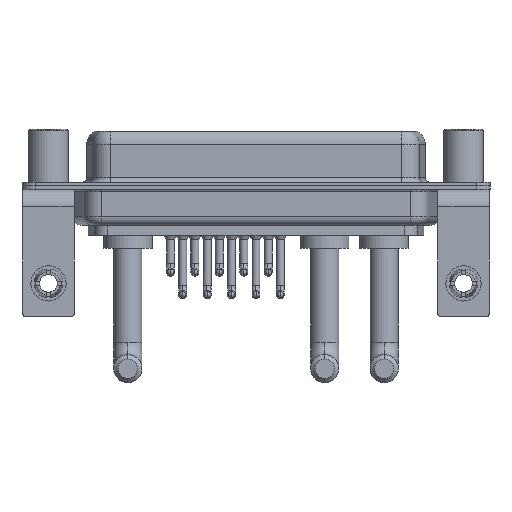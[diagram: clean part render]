
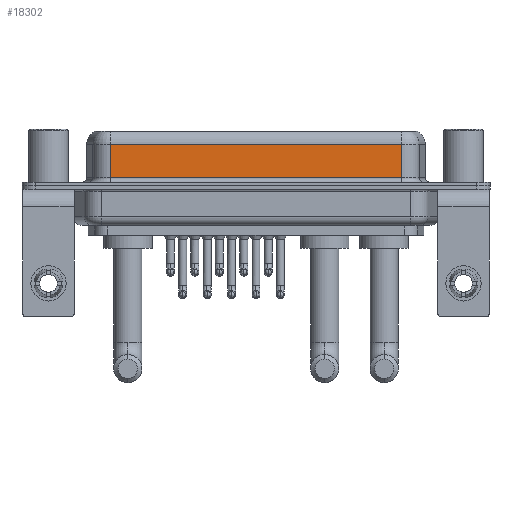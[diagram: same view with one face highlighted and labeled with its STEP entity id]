
A CAD part, front view. The second image highlights one B-rep face of the part: STEP entity #18302.
In plain terms, the highlighted planar face has unit normal (0, -1, 0).
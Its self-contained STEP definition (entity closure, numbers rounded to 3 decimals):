
#898 = EDGE_CURVE ( 'NONE', #4275, #22912, #19926, .T. ) ;
#1198 = FACE_OUTER_BOUND ( 'NONE', #8461, .T. ) ;
#2179 = EDGE_CURVE ( 'NONE', #14506, #22912, #13624, .T. ) ;
#3720 = CARTESIAN_POINT ( 'NONE',  ( 40.037, -3.95, 0.9 ) ) ;
#4275 = VERTEX_POINT ( 'NONE', #19622 ) ;
#4609 = VECTOR ( 'NONE', #14231, 1000. ) ;
#4819 = ORIENTED_EDGE ( 'NONE', *, *, #17110, .T. ) ;
#5041 = DIRECTION ( 'NONE',  ( 0., 0., -1. ) ) ;
#5207 = LINE ( 'NONE', #13895, #4609 ) ;
#5889 = CARTESIAN_POINT ( 'NONE',  ( 40.037, -3.95, 4.65 ) ) ;
#6322 = LINE ( 'NONE', #20639, #19572 ) ;
#6610 = DIRECTION ( 'NONE',  ( 0., 1., 0. ) ) ;
#6916 = DIRECTION ( 'NONE',  ( 1., 0., 0. ) ) ;
#7011 = VERTEX_POINT ( 'NONE', #16318 ) ;
#7277 = EDGE_CURVE ( 'NONE', #14506, #7011, #6322, .T. ) ;
#8328 = VECTOR ( 'NONE', #6916, 1000. ) ;
#8355 = CARTESIAN_POINT ( 'NONE',  ( 40.037, -3.95, 6.4 ) ) ;
#8461 = EDGE_LOOP ( 'NONE', ( #10611, #22834, #4819, #16038 ) ) ;
#10611 = ORIENTED_EDGE ( 'NONE', *, *, #2179, .F. ) ;
#11840 = DIRECTION ( 'NONE',  ( -1., 0., 0. ) ) ;
#13624 = LINE ( 'NONE', #21115, #14077 ) ;
#13895 = CARTESIAN_POINT ( 'NONE',  ( 7.013, -3.95, 6.4 ) ) ;
#14077 = VECTOR ( 'NONE', #5041, 1000. ) ;
#14231 = DIRECTION ( 'NONE',  ( 0., 0., -1. ) ) ;
#14506 = VERTEX_POINT ( 'NONE', #5889 ) ;
#15546 = AXIS2_PLACEMENT_3D ( 'NONE', #8355, #6610, #15631 ) ;
#15631 = DIRECTION ( 'NONE',  ( 0., 0., 1. ) ) ;
#16038 = ORIENTED_EDGE ( 'NONE', *, *, #898, .T. ) ;
#16318 = CARTESIAN_POINT ( 'NONE',  ( 7.013, -3.95, 4.65 ) ) ;
#17110 = EDGE_CURVE ( 'NONE', #7011, #4275, #5207, .T. ) ;
#17606 = CARTESIAN_POINT ( 'NONE',  ( 40.037, -3.95, 0.9 ) ) ;
#18302 = ADVANCED_FACE ( 'NONE', ( #1198 ), #19605, .F. ) ;
#19572 = VECTOR ( 'NONE', #11840, 1000. ) ;
#19605 = PLANE ( 'NONE',  #15546 ) ;
#19622 = CARTESIAN_POINT ( 'NONE',  ( 7.013, -3.95, 0.9 ) ) ;
#19926 = LINE ( 'NONE', #3720, #8328 ) ;
#20639 = CARTESIAN_POINT ( 'NONE',  ( 40.037, -3.95, 4.65 ) ) ;
#21115 = CARTESIAN_POINT ( 'NONE',  ( 40.037, -3.95, 6.4 ) ) ;
#22834 = ORIENTED_EDGE ( 'NONE', *, *, #7277, .T. ) ;
#22912 = VERTEX_POINT ( 'NONE', #17606 ) ;
